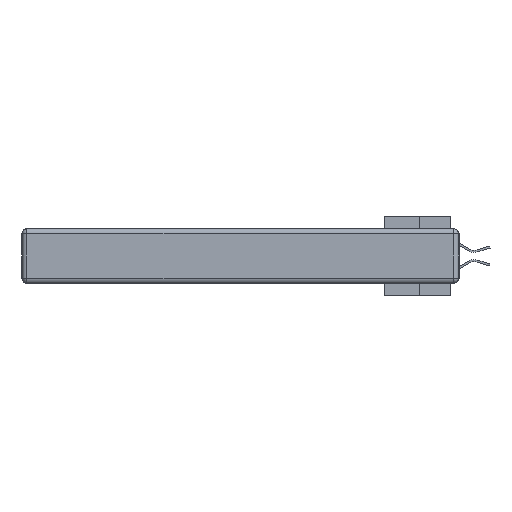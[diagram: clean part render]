
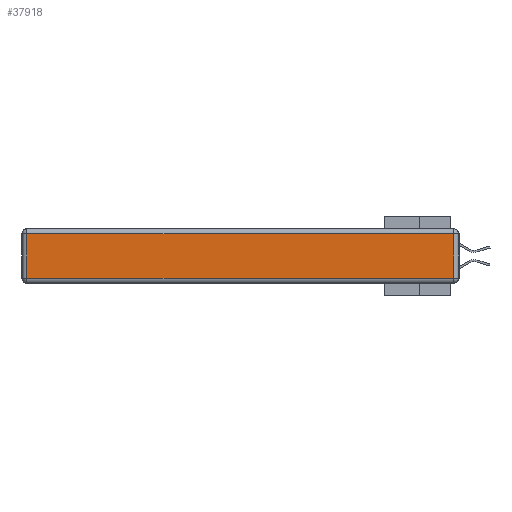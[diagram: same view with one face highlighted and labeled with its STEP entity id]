
A CAD part, left-side view. The second image highlights one B-rep face of the part: STEP entity #37918.
In plain terms, the highlighted planar face has unit normal (-1, 0, 0).
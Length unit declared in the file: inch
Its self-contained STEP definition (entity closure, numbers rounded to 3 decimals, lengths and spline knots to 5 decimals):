
#2215 = CARTESIAN_POINT ( 'NONE',  ( 0., 0., -0.313 ) ) ;
#2416 = CARTESIAN_POINT ( 'NONE',  ( 0., 2.72, -0.03 ) ) ;
#3128 = LINE ( 'NONE', #27261, #35180 ) ;
#4659 = VERTEX_POINT ( 'NONE', #13222 ) ;
#8417 = DIRECTION ( 'NONE',  ( 0., 0., 1. ) ) ;
#8808 = VECTOR ( 'NONE', #12726, 39.37008 ) ;
#10386 = EDGE_CURVE ( 'NONE', #34122, #4659, #15802, .T. ) ;
#12726 = DIRECTION ( 'NONE',  ( 0., 0., -1. ) ) ;
#12859 = VECTOR ( 'NONE', #23961, 39.37008 ) ;
#13222 = CARTESIAN_POINT ( 'NONE',  ( 0., 0.03, -0.313 ) ) ;
#13618 = LINE ( 'NONE', #20612, #16089 ) ;
#15319 = CARTESIAN_POINT ( 'NONE',  ( 0., 2.72, -0.313 ) ) ;
#15802 = LINE ( 'NONE', #2215, #12859 ) ;
#16089 = VECTOR ( 'NONE', #8417, 39.37008 ) ;
#16789 = VERTEX_POINT ( 'NONE', #19628 ) ;
#19628 = CARTESIAN_POINT ( 'NONE',  ( 0., 0.03, -0.03 ) ) ;
#19651 = VERTEX_POINT ( 'NONE', #2416 ) ;
#19910 = ORIENTED_EDGE ( 'NONE', *, *, #33542, .T. ) ;
#20612 = CARTESIAN_POINT ( 'NONE',  ( 0., 0.03, -0.343 ) ) ;
#20747 = EDGE_LOOP ( 'NONE', ( #39797, #28168, #32868, #19910 ) ) ;
#21030 = DIRECTION ( 'NONE',  ( 0., 1., 0. ) ) ;
#22550 = EDGE_CURVE ( 'NONE', #16789, #19651, #3128, .T. ) ;
#23343 = AXIS2_PLACEMENT_3D ( 'NONE', #29205, #35474, #25812 ) ;
#23961 = DIRECTION ( 'NONE',  ( 0., -1., 0. ) ) ;
#25812 = DIRECTION ( 'NONE',  ( 0., 0., 1. ) ) ;
#27261 = CARTESIAN_POINT ( 'NONE',  ( 0., 2.75, -0.03 ) ) ;
#28084 = CARTESIAN_POINT ( 'NONE',  ( 0., 2.72, -0.343 ) ) ;
#28168 = ORIENTED_EDGE ( 'NONE', *, *, #38831, .T. ) ;
#28212 = LINE ( 'NONE', #28084, #8808 ) ;
#28927 = PLANE ( 'NONE',  #23343 ) ;
#29205 = CARTESIAN_POINT ( 'NONE',  ( 0., 0., -0.343 ) ) ;
#32017 = FACE_OUTER_BOUND ( 'NONE', #20747, .T. ) ;
#32868 = ORIENTED_EDGE ( 'NONE', *, *, #22550, .T. ) ;
#33542 = EDGE_CURVE ( 'NONE', #19651, #34122, #28212, .T. ) ;
#34122 = VERTEX_POINT ( 'NONE', #15319 ) ;
#35180 = VECTOR ( 'NONE', #21030, 39.37008 ) ;
#35474 = DIRECTION ( 'NONE',  ( -1., 0., 0. ) ) ;
#37918 = ADVANCED_FACE ( 'NONE', ( #32017 ), #28927, .T. ) ;
#38831 = EDGE_CURVE ( 'NONE', #4659, #16789, #13618, .T. ) ;
#39797 = ORIENTED_EDGE ( 'NONE', *, *, #10386, .T. ) ;
